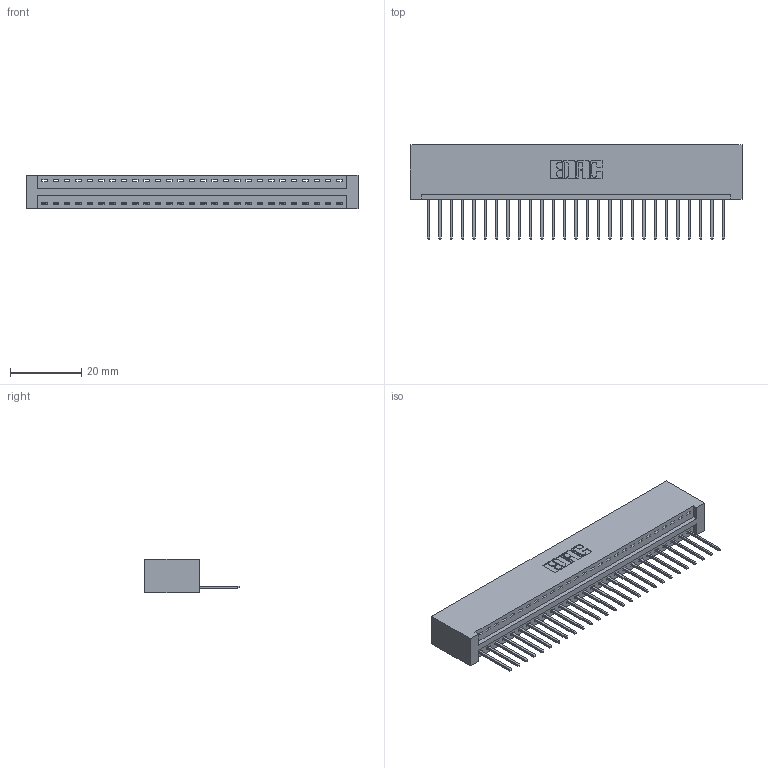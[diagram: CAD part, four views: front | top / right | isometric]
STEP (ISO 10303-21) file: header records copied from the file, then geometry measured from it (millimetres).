
FILE_DESCRIPTION (( 'STEP AP203' ), '1' );
FILE_NAME ('346-027-522-101.STEP', '2018-08-21T23:57:29', ( '' ), ( '' ), 'SwSTEP 2.0', 'SolidWorks 2016', '' );
FILE_SCHEMA (( 'CONFIG_CONTROL_DESIGN' ));
Length unit declared in the file: inch
Products named in the file (3): 346 Part_No Mounting Lugs; 345-292-001_345-293-122; 346-027-522-101
Assembly tree (28 placements, depth 2):
  346-027-522-101
    346 Part_No Mounting Lugs
    345-292-001_345-293-122  x27
Bounding box: 92.96 x 26.42 x 9.4 mm (x, y, z)
Volume: 9348.2 mm3; surface area: 11696.6 mm2
Topology: 28 solids, 28 shells, 1680 faces, 5057 edges, 3334 vertices
Faces by surface type: plane 1152, cylinder 528
Entity records: 18517 total; most frequent: CARTESIAN_POINT 3185, ORIENTED_EDGE 3146, DIRECTION 2823, EDGE_CURVE 1573, LINE 1341, VECTOR 1341, VERTEX_POINT 1046, AXIS2_PLACEMENT_3D 741
